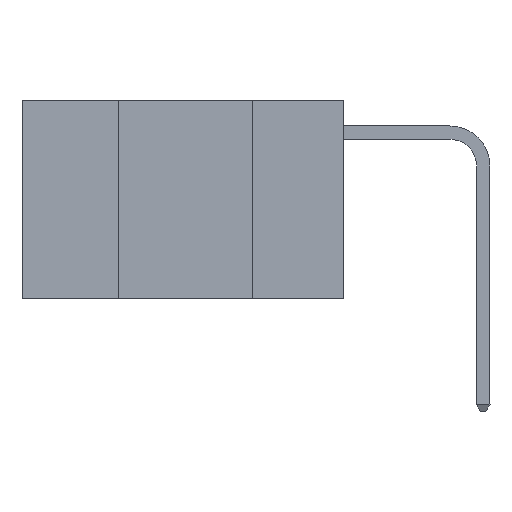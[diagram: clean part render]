
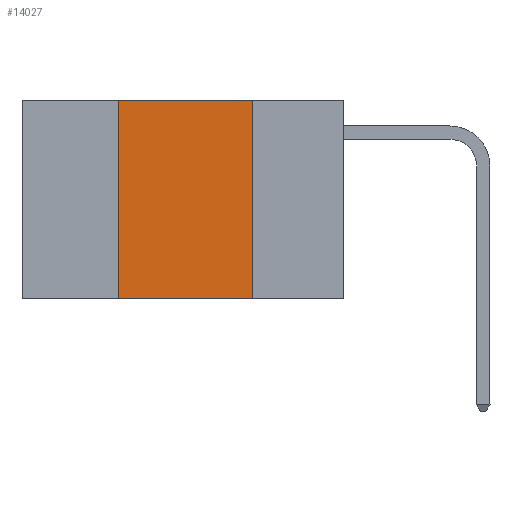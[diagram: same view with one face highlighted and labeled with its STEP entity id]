
A CAD part, left-side view. The second image highlights one B-rep face of the part: STEP entity #14027.
In plain terms, the highlighted planar face has unit normal (-1, 0, 0).
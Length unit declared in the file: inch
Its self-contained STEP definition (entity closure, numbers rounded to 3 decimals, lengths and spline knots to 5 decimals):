
#267 = DIRECTION ( 'NONE',  ( 0., 0., 1. ) ) ;
#446 = EDGE_LOOP ( 'NONE', ( #1225, #20145, #16250, #10644 ) ) ;
#495 = DIRECTION ( 'NONE',  ( 0., -1., 0. ) ) ;
#692 = PLANE ( 'NONE',  #4228 ) ;
#1225 = ORIENTED_EDGE ( 'NONE', *, *, #4633, .F. ) ;
#1275 = CARTESIAN_POINT ( 'NONE',  ( 0., 0.42, -0.37 ) ) ;
#1289 = CARTESIAN_POINT ( 'NONE',  ( 0., 0.17, 0. ) ) ;
#1392 = LINE ( 'NONE', #14166, #19806 ) ;
#1841 = VERTEX_POINT ( 'NONE', #8667 ) ;
#1891 = CARTESIAN_POINT ( 'NONE',  ( 0., 0.17, 0. ) ) ;
#2182 = DIRECTION ( 'NONE',  ( 0., 0., -1. ) ) ;
#2296 = DIRECTION ( 'NONE',  ( 0., 0., -1. ) ) ;
#4228 = AXIS2_PLACEMENT_3D ( 'NONE', #8624, #15061, #2182 ) ;
#4633 = EDGE_CURVE ( 'NONE', #16353, #1841, #10129, .T. ) ;
#5040 = VECTOR ( 'NONE', #495, 39.37008 ) ;
#5774 = FACE_OUTER_BOUND ( 'NONE', #446, .T. ) ;
#5961 = CARTESIAN_POINT ( 'NONE',  ( 0., 0.42, 0. ) ) ;
#6397 = LINE ( 'NONE', #14731, #7561 ) ;
#7561 = VECTOR ( 'NONE', #267, 39.37008 ) ;
#8529 = LINE ( 'NONE', #16661, #5040 ) ;
#8624 = CARTESIAN_POINT ( 'NONE',  ( 0., 0.6, 0. ) ) ;
#8667 = CARTESIAN_POINT ( 'NONE',  ( 0., 0.17, -0.37 ) ) ;
#10129 = LINE ( 'NONE', #1891, #11014 ) ;
#10644 = ORIENTED_EDGE ( 'NONE', *, *, #16357, .T. ) ;
#11014 = VECTOR ( 'NONE', #2296, 39.37008 ) ;
#11144 = EDGE_CURVE ( 'NONE', #12352, #17832, #6397, .T. ) ;
#12352 = VERTEX_POINT ( 'NONE', #1275 ) ;
#13741 = DIRECTION ( 'NONE',  ( 0., -1., 0. ) ) ;
#14027 = ADVANCED_FACE ( 'NONE', ( #5774 ), #692, .F. ) ;
#14166 = CARTESIAN_POINT ( 'NONE',  ( 0., 0.6, -0.37 ) ) ;
#14731 = CARTESIAN_POINT ( 'NONE',  ( 0., 0.42, 0. ) ) ;
#15061 = DIRECTION ( 'NONE',  ( 1., 0., 0. ) ) ;
#16250 = ORIENTED_EDGE ( 'NONE', *, *, #11144, .F. ) ;
#16353 = VERTEX_POINT ( 'NONE', #1289 ) ;
#16357 = EDGE_CURVE ( 'NONE', #12352, #1841, #1392, .T. ) ;
#16661 = CARTESIAN_POINT ( 'NONE',  ( 0., 0.6, 0. ) ) ;
#17832 = VERTEX_POINT ( 'NONE', #5961 ) ;
#19806 = VECTOR ( 'NONE', #13741, 39.37008 ) ;
#20145 = ORIENTED_EDGE ( 'NONE', *, *, #20207, .F. ) ;
#20207 = EDGE_CURVE ( 'NONE', #17832, #16353, #8529, .T. ) ;
